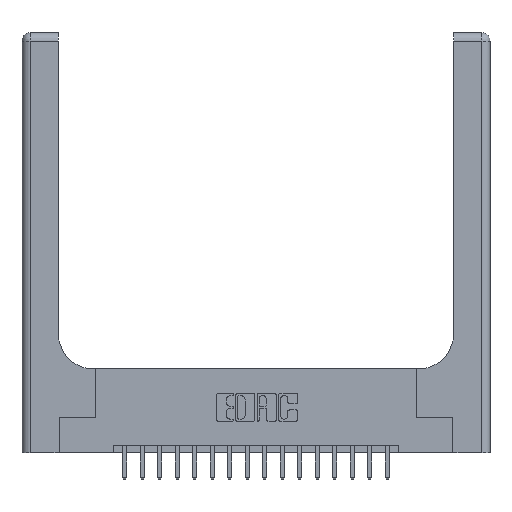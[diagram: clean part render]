
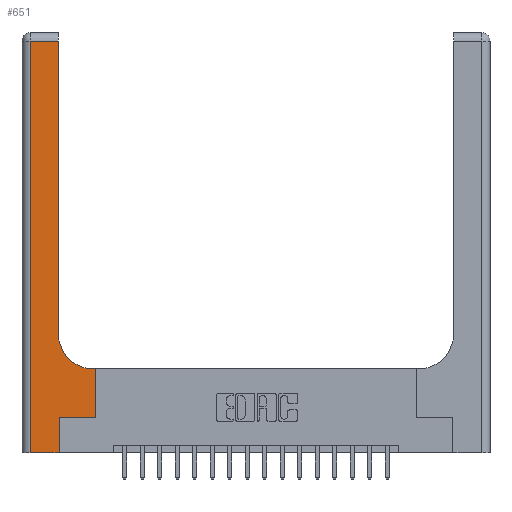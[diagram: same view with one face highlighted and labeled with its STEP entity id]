
A CAD part, top view. The second image highlights one B-rep face of the part: STEP entity #651.
In plain terms, the highlighted planar face has unit normal (0, 0, 1).
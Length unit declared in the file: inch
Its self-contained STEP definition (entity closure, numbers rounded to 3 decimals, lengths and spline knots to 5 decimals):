
#651 = ADVANCED_FACE ( 'NONE', ( #3652 ), #15707, .F. ) ;
#1047 = AXIS2_PLACEMENT_3D ( 'NONE', #12808, #5452, #17211 ) ;
#1129 = EDGE_CURVE ( 'NONE', #1155, #1137, #4103, .T. ) ;
#1137 = VERTEX_POINT ( 'NONE', #2619 ) ;
#1155 = VERTEX_POINT ( 'NONE', #3632 ) ;
#1217 = VERTEX_POINT ( 'NONE', #12781 ) ;
#1258 = EDGE_CURVE ( 'NONE', #18576, #15873, #1433, .T. ) ;
#1289 = EDGE_CURVE ( 'NONE', #15873, #10820, #15064, .T. ) ;
#1433 = LINE ( 'NONE', #5804, #9425 ) ;
#1846 = CARTESIAN_POINT ( 'NONE',  ( 0.51, 0.85, 0.37 ) ) ;
#2431 = VECTOR ( 'NONE', #8992, 39.37008 ) ;
#2522 = CARTESIAN_POINT ( 'NONE',  ( 0.51, 0.6, 0.37 ) ) ;
#2587 = CARTESIAN_POINT ( 'NONE',  ( 0.06, 3., 0.37 ) ) ;
#2619 = CARTESIAN_POINT ( 'NONE',  ( 0.26, 2.94, 0.37 ) ) ;
#2853 = CARTESIAN_POINT ( 'NONE',  ( 0., 0., 0.37 ) ) ;
#3485 = EDGE_CURVE ( 'NONE', #17883, #11443, #13023, .T. ) ;
#3632 = CARTESIAN_POINT ( 'NONE',  ( 0.26, 0.85, 0.37 ) ) ;
#3652 = FACE_OUTER_BOUND ( 'NONE', #5121, .T. ) ;
#4064 = CARTESIAN_POINT ( 'NONE',  ( 0.265, 0., 0.37 ) ) ;
#4103 = LINE ( 'NONE', #18691, #10704 ) ;
#4488 = LINE ( 'NONE', #14638, #13992 ) ;
#4787 = DIRECTION ( 'NONE',  ( -1., 0., 0. ) ) ;
#4813 = ORIENTED_EDGE ( 'NONE', *, *, #3485, .T. ) ;
#5121 = EDGE_LOOP ( 'NONE', ( #12972, #8455, #4813, #8499, #16574, #16010, #6990, #11752, #9807 ) ) ;
#5168 = VECTOR ( 'NONE', #18296, 39.37008 ) ;
#5307 = CIRCLE ( 'NONE', #18342, 0.25 ) ;
#5452 = DIRECTION ( 'NONE',  ( 0., 0., -1. ) ) ;
#5537 = VECTOR ( 'NONE', #4787, 39.37008 ) ;
#5804 = CARTESIAN_POINT ( 'NONE',  ( 0.265, 0., 0.37 ) ) ;
#6220 = DIRECTION ( 'NONE',  ( 0., 0., -1. ) ) ;
#6800 = EDGE_CURVE ( 'NONE', #10820, #1217, #4488, .T. ) ;
#6990 = ORIENTED_EDGE ( 'NONE', *, *, #6800, .T. ) ;
#7446 = CARTESIAN_POINT ( 'NONE',  ( 0.265, 0.25, 0.37 ) ) ;
#7915 = DIRECTION ( 'NONE',  ( 1., 0., 0. ) ) ;
#7932 = DIRECTION ( 'NONE',  ( -1., 0., 0. ) ) ;
#8226 = VECTOR ( 'NONE', #17530, 39.37008 ) ;
#8455 = ORIENTED_EDGE ( 'NONE', *, *, #13942, .T. ) ;
#8499 = ORIENTED_EDGE ( 'NONE', *, *, #8923, .T. ) ;
#8923 = EDGE_CURVE ( 'NONE', #11443, #18576, #13398, .T. ) ;
#8992 = DIRECTION ( 'NONE',  ( 1., 0., 0. ) ) ;
#9425 = VECTOR ( 'NONE', #11780, 39.37008 ) ;
#9435 = LINE ( 'NONE', #15498, #15742 ) ;
#9807 = ORIENTED_EDGE ( 'NONE', *, *, #15986, .T. ) ;
#10566 = CARTESIAN_POINT ( 'NONE',  ( 0.26, 0.6, 0.37 ) ) ;
#10585 = CARTESIAN_POINT ( 'NONE',  ( 0.06, 2.94, 0.37 ) ) ;
#10704 = VECTOR ( 'NONE', #17387, 39.37008 ) ;
#10751 = LINE ( 'NONE', #10566, #5537 ) ;
#10820 = VERTEX_POINT ( 'NONE', #12854 ) ;
#11443 = VERTEX_POINT ( 'NONE', #13541 ) ;
#11752 = ORIENTED_EDGE ( 'NONE', *, *, #12598, .T. ) ;
#11780 = DIRECTION ( 'NONE',  ( 0., 1., 0. ) ) ;
#12077 = VERTEX_POINT ( 'NONE', #2522 ) ;
#12598 = EDGE_CURVE ( 'NONE', #1217, #12077, #10751, .T. ) ;
#12781 = CARTESIAN_POINT ( 'NONE',  ( 0.528, 0.6, 0.37 ) ) ;
#12808 = CARTESIAN_POINT ( 'NONE',  ( 0., 3., 0.37 ) ) ;
#12854 = CARTESIAN_POINT ( 'NONE',  ( 0.528, 0.25, 0.37 ) ) ;
#12972 = ORIENTED_EDGE ( 'NONE', *, *, #1129, .T. ) ;
#13023 = LINE ( 'NONE', #2587, #8226 ) ;
#13398 = LINE ( 'NONE', #2853, #5168 ) ;
#13541 = CARTESIAN_POINT ( 'NONE',  ( 0.06, 0., 0.37 ) ) ;
#13942 = EDGE_CURVE ( 'NONE', #1137, #17883, #9435, .T. ) ;
#13992 = VECTOR ( 'NONE', #19249, 39.37008 ) ;
#14638 = CARTESIAN_POINT ( 'NONE',  ( 0.528, 0.25, 0.37 ) ) ;
#15064 = LINE ( 'NONE', #17974, #2431 ) ;
#15498 = CARTESIAN_POINT ( 'NONE',  ( 0., 2.94, 0.37 ) ) ;
#15707 = PLANE ( 'NONE',  #1047 ) ;
#15742 = VECTOR ( 'NONE', #7932, 39.37008 ) ;
#15873 = VERTEX_POINT ( 'NONE', #7446 ) ;
#15986 = EDGE_CURVE ( 'NONE', #12077, #1155, #5307, .T. ) ;
#16010 = ORIENTED_EDGE ( 'NONE', *, *, #1289, .T. ) ;
#16574 = ORIENTED_EDGE ( 'NONE', *, *, #1258, .T. ) ;
#17211 = DIRECTION ( 'NONE',  ( -1., 0., 0. ) ) ;
#17387 = DIRECTION ( 'NONE',  ( 0., 1., 0. ) ) ;
#17530 = DIRECTION ( 'NONE',  ( 0., -1., 0. ) ) ;
#17883 = VERTEX_POINT ( 'NONE', #10585 ) ;
#17974 = CARTESIAN_POINT ( 'NONE',  ( 0.265, 0.25, 0.37 ) ) ;
#18296 = DIRECTION ( 'NONE',  ( 1., 0., 0. ) ) ;
#18342 = AXIS2_PLACEMENT_3D ( 'NONE', #1846, #6220, #7915 ) ;
#18576 = VERTEX_POINT ( 'NONE', #4064 ) ;
#18691 = CARTESIAN_POINT ( 'NONE',  ( 0.26, 3., 0.37 ) ) ;
#19249 = DIRECTION ( 'NONE',  ( 0., 1., 0. ) ) ;
